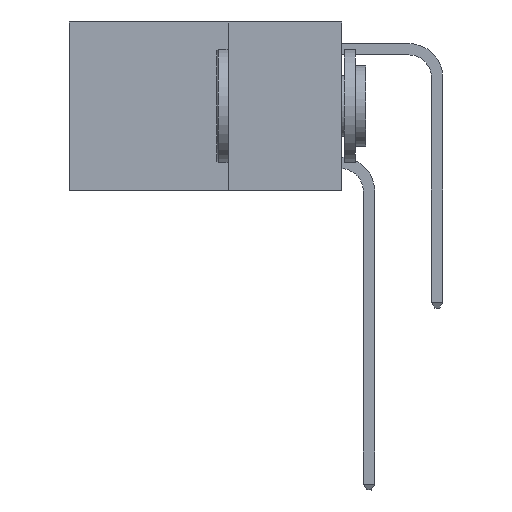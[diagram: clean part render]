
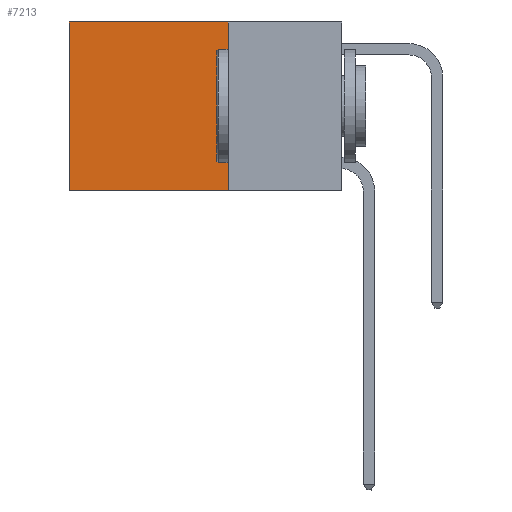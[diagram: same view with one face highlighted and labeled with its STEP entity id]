
A CAD part, left-side view. The second image highlights one B-rep face of the part: STEP entity #7213.
In plain terms, the highlighted planar face has unit normal (-1, 0, 0).
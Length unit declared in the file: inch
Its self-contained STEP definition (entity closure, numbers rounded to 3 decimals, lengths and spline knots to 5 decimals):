
#1131 = CARTESIAN_POINT ( 'NONE',  ( 0.2625, 0.25, 0. ) ) ;
#1598 = DIRECTION ( 'NONE',  ( 0., 1., 0. ) ) ;
#3186 = DIRECTION ( 'NONE',  ( 0., 0., -1. ) ) ;
#3486 = LINE ( 'NONE', #3599, #5803 ) ;
#3599 = CARTESIAN_POINT ( 'NONE',  ( 0.2625, 0.25, -0.37 ) ) ;
#3627 = EDGE_CURVE ( 'NONE', #3674, #20653, #3486, .T. ) ;
#3674 = VERTEX_POINT ( 'NONE', #19367 ) ;
#4667 = VERTEX_POINT ( 'NONE', #11971 ) ;
#4684 = DIRECTION ( 'NONE',  ( 0., 0., -1. ) ) ;
#4948 = EDGE_CURVE ( 'NONE', #19679, #4667, #15691, .T. ) ;
#5803 = VECTOR ( 'NONE', #7594, 39.37008 ) ;
#6535 = EDGE_CURVE ( 'NONE', #4667, #20653, #8357, .T. ) ;
#6600 = CARTESIAN_POINT ( 'NONE',  ( 0.2625, 0.6, -0.37 ) ) ;
#7213 = ADVANCED_FACE ( 'NONE', ( #12900 ), #7292, .F. ) ;
#7292 = PLANE ( 'NONE',  #17904 ) ;
#7594 = DIRECTION ( 'NONE',  ( 0., 1., 0. ) ) ;
#8357 = LINE ( 'NONE', #24324, #13079 ) ;
#9249 = EDGE_CURVE ( 'NONE', #19679, #3674, #19665, .T. ) ;
#9774 = VECTOR ( 'NONE', #4684, 39.37008 ) ;
#10169 = CARTESIAN_POINT ( 'NONE',  ( 0.2625, 0.25, 0. ) ) ;
#11250 = ORIENTED_EDGE ( 'NONE', *, *, #3627, .F. ) ;
#11971 = CARTESIAN_POINT ( 'NONE',  ( 0.2625, 0.6, 0. ) ) ;
#12900 = FACE_OUTER_BOUND ( 'NONE', #15397, .T. ) ;
#13079 = VECTOR ( 'NONE', #14311, 39.37008 ) ;
#13271 = ORIENTED_EDGE ( 'NONE', *, *, #9249, .F. ) ;
#14311 = DIRECTION ( 'NONE',  ( 0., 0., -1. ) ) ;
#14945 = ORIENTED_EDGE ( 'NONE', *, *, #4948, .T. ) ;
#15037 = DIRECTION ( 'NONE',  ( 1., 0., 0. ) ) ;
#15397 = EDGE_LOOP ( 'NONE', ( #22438, #11250, #13271, #14945 ) ) ;
#15691 = LINE ( 'NONE', #19026, #15839 ) ;
#15839 = VECTOR ( 'NONE', #1598, 39.37008 ) ;
#16931 = CARTESIAN_POINT ( 'NONE',  ( 0.2625, 0.25, 0. ) ) ;
#17904 = AXIS2_PLACEMENT_3D ( 'NONE', #16931, #15037, #3186 ) ;
#19026 = CARTESIAN_POINT ( 'NONE',  ( 0.2625, 0.25, 0. ) ) ;
#19367 = CARTESIAN_POINT ( 'NONE',  ( 0.2625, 0.25, -0.37 ) ) ;
#19665 = LINE ( 'NONE', #10169, #9774 ) ;
#19679 = VERTEX_POINT ( 'NONE', #1131 ) ;
#20653 = VERTEX_POINT ( 'NONE', #6600 ) ;
#22438 = ORIENTED_EDGE ( 'NONE', *, *, #6535, .T. ) ;
#24324 = CARTESIAN_POINT ( 'NONE',  ( 0.2625, 0.6, 0. ) ) ;
